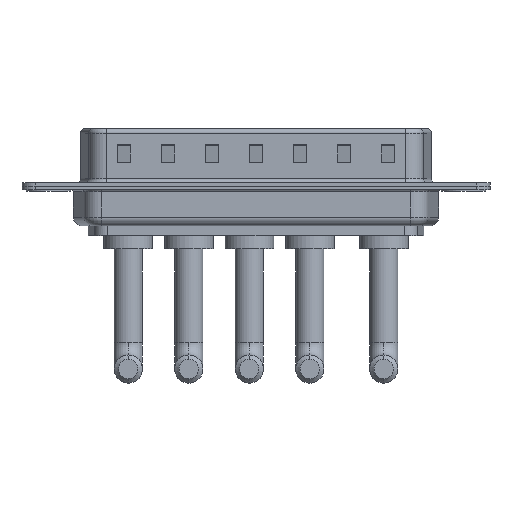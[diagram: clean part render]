
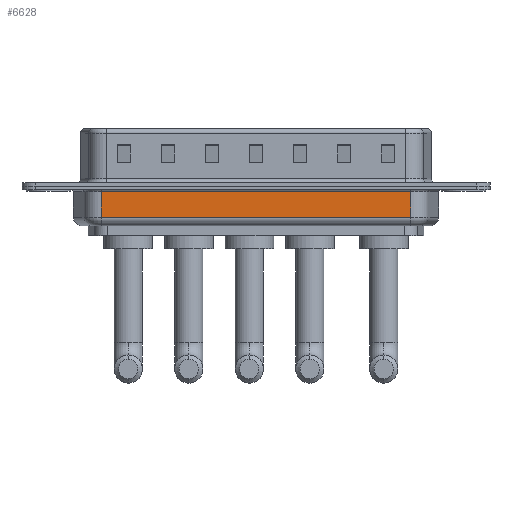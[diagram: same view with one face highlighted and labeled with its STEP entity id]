
A CAD part, front view. The second image highlights one B-rep face of the part: STEP entity #6628.
In plain terms, the highlighted planar face has unit normal (0, -1, 0).
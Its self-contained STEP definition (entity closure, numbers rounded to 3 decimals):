
#102 = FACE_OUTER_BOUND ( 'NONE', #1430, .T. ) ;
#1241 = VECTOR ( 'NONE', #4262, 1000. ) ;
#1246 = VECTOR ( 'NONE', #1266, 1000. ) ;
#1266 = DIRECTION ( 'NONE',  ( 0., 0., 1. ) ) ;
#1430 = EDGE_LOOP ( 'NONE', ( #11620, #8282, #5351, #8297 ) ) ;
#1657 = LINE ( 'NONE', #5515, #5422 ) ;
#2060 = CARTESIAN_POINT ( 'NONE',  ( 41.044, -5.35, -0.65 ) ) ;
#2663 = VECTOR ( 'NONE', #3390, 1000. ) ;
#2709 = VERTEX_POINT ( 'NONE', #2060 ) ;
#2814 = CARTESIAN_POINT ( 'NONE',  ( 6.006, -5.35, -3.5 ) ) ;
#2971 = VERTEX_POINT ( 'NONE', #2814 ) ;
#3390 = DIRECTION ( 'NONE',  ( -1., 0., 0. ) ) ;
#3418 = CARTESIAN_POINT ( 'NONE',  ( 41.044, -5.35, -3.5 ) ) ;
#4131 = DIRECTION ( 'NONE',  ( 0., 1., 0. ) ) ;
#4227 = CARTESIAN_POINT ( 'NONE',  ( 6.006, -5.35, -0.65 ) ) ;
#4262 = DIRECTION ( 'NONE',  ( 0., 0., 1. ) ) ;
#5268 = LINE ( 'NONE', #9153, #1241 ) ;
#5351 = ORIENTED_EDGE ( 'NONE', *, *, #7734, .T. ) ;
#5422 = VECTOR ( 'NONE', #11332, 1000. ) ;
#5515 = CARTESIAN_POINT ( 'NONE',  ( 6.006, -5.35, -3.5 ) ) ;
#5887 = CARTESIAN_POINT ( 'NONE',  ( 6.006, -5.35, -4.5 ) ) ;
#6523 = EDGE_CURVE ( 'NONE', #2971, #6772, #1657, .T. ) ;
#6628 = ADVANCED_FACE ( 'NONE', ( #102 ), #8881, .F. ) ;
#6772 = VERTEX_POINT ( 'NONE', #3418 ) ;
#7316 = EDGE_CURVE ( 'NONE', #2709, #11357, #11350, .T. ) ;
#7734 = EDGE_CURVE ( 'NONE', #6772, #2709, #5268, .T. ) ;
#8123 = LINE ( 'NONE', #10940, #1246 ) ;
#8282 = ORIENTED_EDGE ( 'NONE', *, *, #6523, .T. ) ;
#8297 = ORIENTED_EDGE ( 'NONE', *, *, #7316, .T. ) ;
#8881 = PLANE ( 'NONE',  #10334 ) ;
#9153 = CARTESIAN_POINT ( 'NONE',  ( 41.044, -5.35, -4.5 ) ) ;
#9351 = CARTESIAN_POINT ( 'NONE',  ( 6.006, -5.35, -0.65 ) ) ;
#10334 = AXIS2_PLACEMENT_3D ( 'NONE', #5887, #4131, #10736 ) ;
#10496 = EDGE_CURVE ( 'NONE', #2971, #11357, #8123, .T. ) ;
#10736 = DIRECTION ( 'NONE',  ( 0., 0., 1. ) ) ;
#10940 = CARTESIAN_POINT ( 'NONE',  ( 6.006, -5.35, -4.5 ) ) ;
#11332 = DIRECTION ( 'NONE',  ( 1., 0., 0. ) ) ;
#11350 = LINE ( 'NONE', #9351, #2663 ) ;
#11357 = VERTEX_POINT ( 'NONE', #4227 ) ;
#11620 = ORIENTED_EDGE ( 'NONE', *, *, #10496, .F. ) ;
